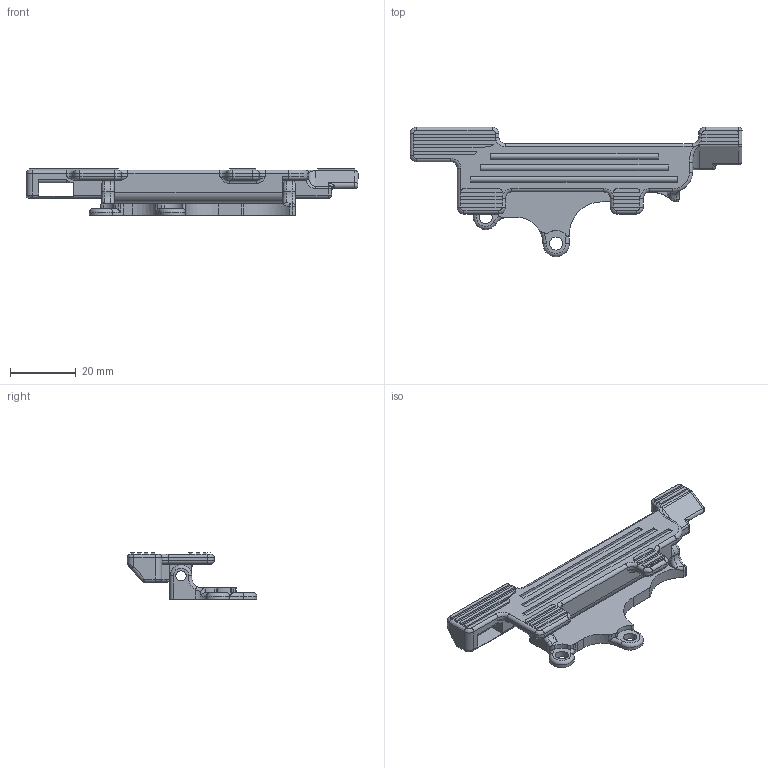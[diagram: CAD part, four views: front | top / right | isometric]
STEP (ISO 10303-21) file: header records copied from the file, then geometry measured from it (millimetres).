
FILE_DESCRIPTION(/* description */ (''),/* implementation_level */ '2;1');
FILE_NAME(/* name */ 'The Peace Release.step',/* time_stamp */ '2022-05-23T12:14:06-04:00',/* author */ (''),/* organization */ (''),/* preprocessor_version */ 'ST-DEVELOPER v18.1',/* originating_system */ 'Autodesk Translation Framework v10.14.0.1471',/* authorisation */ '');
FILE_SCHEMA (('AUTOMOTIVE_DESIGN { 1 0 10303 214 3 1 1 }'));
Length unit declared in the file: millimetre
Products named in the file (3): WRAITH; ARK2.0; The Peace Release
Assembly tree (2 placements, depth 3):
  WRAITH
    ARK2.0
      The Peace Release
Bounding box: 100.97 x 39.35 x 14.22 mm (x, y, z)
Volume: 12718.2 mm3; surface area: 10082.6 mm2
Topology: 5 solids, 5 shells, 369 faces, 892 edges, 531 vertices
Faces by surface type: plane 169, cylinder 130, bspline 31, torus 29, sphere 10
Full cylindrical faces by diameter (mm): 1.75 x9, 3.1 x3, 3.962 x2
Entity records: 11522 total; most frequent: CARTESIAN_POINT 2812, DIRECTION 1855, ORIENTED_EDGE 1774, EDGE_CURVE 887, AXIS2_PLACEMENT_3D 675, VERTEX_POINT 531, LINE 505, VECTOR 505
